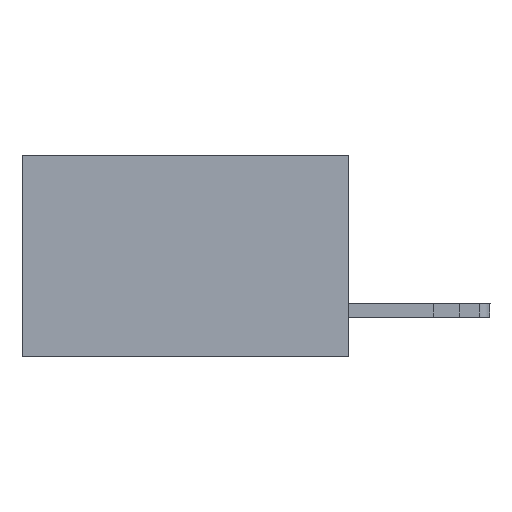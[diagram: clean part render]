
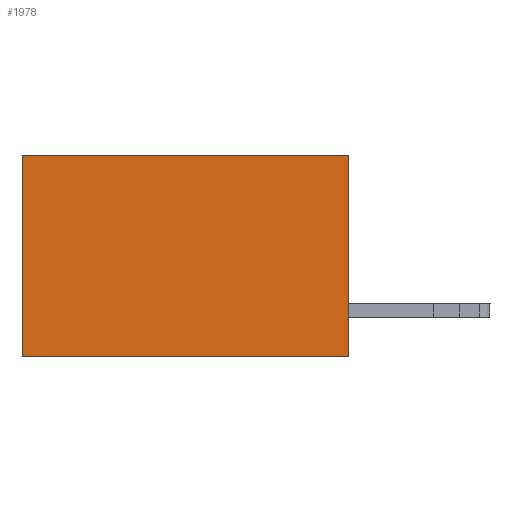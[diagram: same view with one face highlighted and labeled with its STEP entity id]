
A CAD part, left-side view. The second image highlights one B-rep face of the part: STEP entity #1978.
In plain terms, the highlighted planar face has unit normal (-1, 0, 0).
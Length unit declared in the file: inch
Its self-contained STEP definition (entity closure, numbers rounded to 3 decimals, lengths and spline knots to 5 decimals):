
#473 = EDGE_LOOP ( 'NONE', ( #1435, #5118, #1691, #1813 ) ) ;
#664 = CARTESIAN_POINT ( 'NONE',  ( 0.2615, 0.6, -0.37 ) ) ;
#996 = VECTOR ( 'NONE', #6707, 39.37008 ) ;
#1435 = ORIENTED_EDGE ( 'NONE', *, *, #9673, .T. ) ;
#1691 = ORIENTED_EDGE ( 'NONE', *, *, #8624, .F. ) ;
#1813 = ORIENTED_EDGE ( 'NONE', *, *, #8886, .T. ) ;
#1819 = DIRECTION ( 'NONE',  ( 0., 0., -1. ) ) ;
#1978 = ADVANCED_FACE ( 'NONE', ( #8939 ), #8853, .F. ) ;
#2400 = DIRECTION ( 'NONE',  ( 0., 0., -1. ) ) ;
#3162 = CARTESIAN_POINT ( 'NONE',  ( 0.2615, 0.6, 0. ) ) ;
#3787 = CARTESIAN_POINT ( 'NONE',  ( 0.2615, 0., -0.37 ) ) ;
#4668 = LINE ( 'NONE', #10098, #7221 ) ;
#5118 = ORIENTED_EDGE ( 'NONE', *, *, #9176, .F. ) ;
#5553 = VERTEX_POINT ( 'NONE', #3787 ) ;
#6002 = DIRECTION ( 'NONE',  ( 1., 0., 0. ) ) ;
#6707 = DIRECTION ( 'NONE',  ( 0., 1., 0. ) ) ;
#7146 = VERTEX_POINT ( 'NONE', #3162 ) ;
#7221 = VECTOR ( 'NONE', #2400, 39.37008 ) ;
#7375 = CARTESIAN_POINT ( 'NONE',  ( 0.2615, 0., -0.37 ) ) ;
#7427 = LINE ( 'NONE', #7375, #12823 ) ;
#7604 = AXIS2_PLACEMENT_3D ( 'NONE', #12913, #6002, #8706 ) ;
#8272 = VECTOR ( 'NONE', #11528, 39.37008 ) ;
#8624 = EDGE_CURVE ( 'NONE', #10312, #5553, #7427, .T. ) ;
#8706 = DIRECTION ( 'NONE',  ( 0., 0., -1. ) ) ;
#8853 = PLANE ( 'NONE',  #7604 ) ;
#8886 = EDGE_CURVE ( 'NONE', #10312, #7146, #12648, .T. ) ;
#8939 = FACE_OUTER_BOUND ( 'NONE', #473, .T. ) ;
#9176 = EDGE_CURVE ( 'NONE', #5553, #12112, #11483, .T. ) ;
#9673 = EDGE_CURVE ( 'NONE', #7146, #12112, #4668, .T. ) ;
#10098 = CARTESIAN_POINT ( 'NONE',  ( 0.2615, 0.6, -0.37 ) ) ;
#10312 = VERTEX_POINT ( 'NONE', #13627 ) ;
#11483 = LINE ( 'NONE', #13626, #8272 ) ;
#11528 = DIRECTION ( 'NONE',  ( 0., 1., 0. ) ) ;
#12090 = CARTESIAN_POINT ( 'NONE',  ( 0.2615, 0., 0. ) ) ;
#12112 = VERTEX_POINT ( 'NONE', #664 ) ;
#12648 = LINE ( 'NONE', #12090, #996 ) ;
#12823 = VECTOR ( 'NONE', #1819, 39.37008 ) ;
#12913 = CARTESIAN_POINT ( 'NONE',  ( 0.2615, 0., -0.37 ) ) ;
#13626 = CARTESIAN_POINT ( 'NONE',  ( 0.2615, 0., -0.37 ) ) ;
#13627 = CARTESIAN_POINT ( 'NONE',  ( 0.2615, 0., 0. ) ) ;
